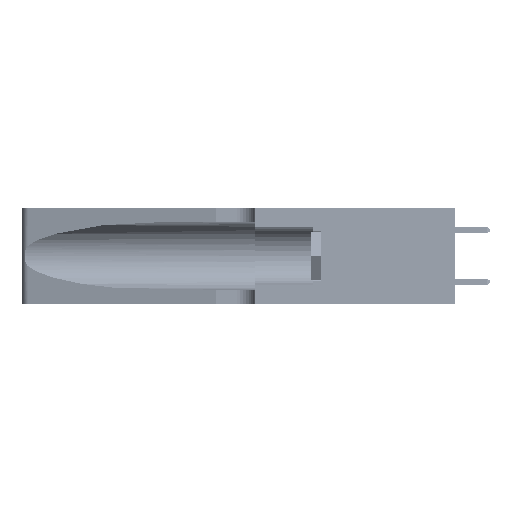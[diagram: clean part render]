
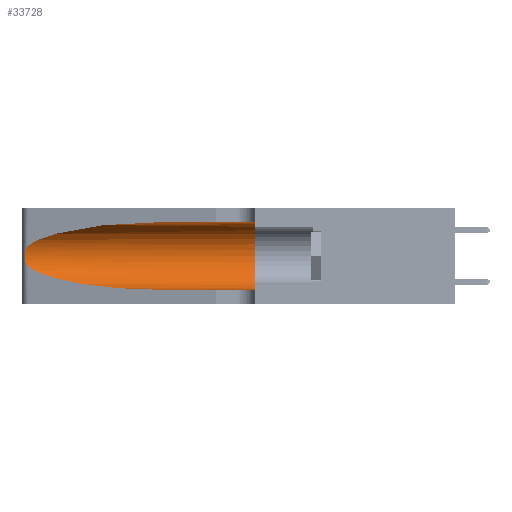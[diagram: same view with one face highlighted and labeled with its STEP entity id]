
A CAD part, left-side view. The second image highlights one B-rep face of the part: STEP entity #33728.
In plain terms, the highlighted cylindrical face has radius 3.308 mm (diameter 6.617 mm), a partial arc.
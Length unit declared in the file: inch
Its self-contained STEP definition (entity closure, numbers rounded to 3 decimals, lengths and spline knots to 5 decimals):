
#523 = VERTEX_POINT ( 'NONE', #7090 ) ;
#2039 = VERTEX_POINT ( 'NONE', #13384 ) ;
#2302 = VERTEX_POINT ( 'NONE', #48875 ) ;
#2403 = VECTOR ( 'NONE', #39100, 39.37008 ) ;
#3396 = LINE ( 'NONE', #21980, #17135 ) ;
#3776 = ORIENTED_EDGE ( 'NONE', *, *, #5392, .T. ) ;
#4815 = CYLINDRICAL_SURFACE ( 'NONE', #41524, 0.13025 ) ;
#5392 = EDGE_CURVE ( 'NONE', #2302, #32435, #41210, .T. ) ;
#6046 = CARTESIAN_POINT ( 'NONE',  ( 0.25639, 1.23186, 0.15144 ) ) ;
#7090 = CARTESIAN_POINT ( 'NONE',  ( 0.1305, 0.35, 0.31525 ) ) ;
#7430 = FACE_OUTER_BOUND ( 'NONE', #9912, .T. ) ;
#9493 = DIRECTION ( 'NONE',  ( 0., 1., 0. ) ) ;
#9912 = EDGE_LOOP ( 'NONE', ( #3776, #40965, #29007, #22652, #28667, #22535 ) ) ;
#10373 = CARTESIAN_POINT ( 'NONE',  ( 0.25639, 1.23184, 0.21858 ) ) ;
#11525 = CARTESIAN_POINT ( 'NONE',  ( 0.1305, 1.61858, 0.185 ) ) ;
#13384 = CARTESIAN_POINT ( 'NONE',  ( 0.25487, 1.22718, 0.14631 ) ) ;
#14968 = VERTEX_POINT ( 'NONE', #16529 ) ;
#15858 = CARTESIAN_POINT ( 'NONE',  ( 0.25487, 1.22718, 0.22369 ) ) ;
#16148 = DIRECTION ( 'NONE',  ( 0., 0., -1. ) ) ;
#16529 = CARTESIAN_POINT ( 'NONE',  ( 0.1305, 0.72297, 0.05475 ) ) ;
#17135 = VECTOR ( 'NONE', #51226, 39.37008 ) ;
#18292 = CARTESIAN_POINT ( 'NONE',  ( 0.25787, 1.23484, 0.2124 ) ) ;
#19939 = CIRCLE ( 'NONE', #35806, 0.13025 ) ;
#20178 = DIRECTION ( 'NONE',  ( 0., -1., 0. ) ) ;
#20579 = EDGE_CURVE ( 'NONE', #523, #42162, #19939, .T. ) ;
#21980 = CARTESIAN_POINT ( 'NONE',  ( 0.1305, 1.61858, 0.05475 ) ) ;
#22315 = CARTESIAN_POINT ( 'NONE',  ( 0.26018, 1.23835, 0.19895 ) ) ;
#22503 = CARTESIAN_POINT ( 'NONE',  ( 0.26017, 1.23833, 0.17102 ) ) ;
#22535 = ORIENTED_EDGE ( 'NONE', *, *, #44434, .F. ) ;
#22652 = ORIENTED_EDGE ( 'NONE', *, *, #53370, .T. ) ;
#23007 = CARTESIAN_POINT ( 'NONE',  ( 0.1305, 1.61858, 0.31525 ) ) ;
#24671 = CARTESIAN_POINT ( 'NONE',  ( 0.2373, 1.15595, 0.28018 ) ) ;
#24755 = CARTESIAN_POINT ( 'NONE',  ( 0.1305, 0.72297, 0.05475 ) ) ;
#25222 = CARTESIAN_POINT ( 'NONE',  ( 0.25487, 1.22718, 0.22369 ) ) ;
#26155 = CARTESIAN_POINT ( 'NONE',  ( 0.1305, 0.35, 0.185 ) ) ;
#26869 = CARTESIAN_POINT ( 'NONE',  ( 0.25856, 1.23593, 0.16098 ) ) ;
#28667 = ORIENTED_EDGE ( 'NONE', *, *, #20579, .F. ) ;
#29007 = ORIENTED_EDGE ( 'NONE', *, *, #31150, .T. ) ;
#31076 = CARTESIAN_POINT ( 'NONE',  ( 0.26075, 1.23896, 0.178 ) ) ;
#31150 = EDGE_CURVE ( 'NONE', #2039, #14968, #37190, .T. ) ;
#32435 = VERTEX_POINT ( 'NONE', #15858 ) ;
#33110 = CARTESIAN_POINT ( 'NONE',  ( 0.18966, 0.96281, 0.31525 ) ) ;
#33645 = CARTESIAN_POINT ( 'NONE',  ( 0.1305, 0.72297, 0.31525 ) ) ;
#33728 = ADVANCED_FACE ( 'NONE', ( #7430 ), #4815, .F. ) ;
#34932 = CARTESIAN_POINT ( 'NONE',  ( 0.25854, 1.2359, 0.20912 ) ) ;
#35287 = CARTESIAN_POINT ( 'NONE',  ( 0.25555, 1.22993, 0.14849 ) ) ;
#35806 = AXIS2_PLACEMENT_3D ( 'NONE', #26155, #9493, #38766 ) ;
#37190 =( BOUNDED_CURVE ( )  B_SPLINE_CURVE ( 3, ( #37193, #41573, #53659, #24755 ),
 .UNSPECIFIED., .F., .F. ) 
 B_SPLINE_CURVE_WITH_KNOTS ( ( 4, 4 ),
 ( 3.44316, 4.71239 ),
 .UNSPECIFIED. ) 
 CURVE ( )  GEOMETRIC_REPRESENTATION_ITEM ( )  RATIONAL_B_SPLINE_CURVE ( ( 1., 0.87, 0.87, 1. ) ) 
 REPRESENTATION_ITEM ( '' )  );
#37193 = CARTESIAN_POINT ( 'NONE',  ( 0.25487, 1.22718, 0.14631 ) ) ;
#38418 = EDGE_CURVE ( 'NONE', #32435, #2039, #42881, .T. ) ;
#38766 = DIRECTION ( 'NONE',  ( 0., 0., 1. ) ) ;
#39100 = DIRECTION ( 'NONE',  ( 0., -1., 0. ) ) ;
#40965 = ORIENTED_EDGE ( 'NONE', *, *, #38418, .T. ) ;
#41210 =( BOUNDED_CURVE ( )  B_SPLINE_CURVE ( 3, ( #33645, #33110, #24671, #25222 ),
 .UNSPECIFIED., .F., .F. ) 
 B_SPLINE_CURVE_WITH_KNOTS ( ( 4, 4 ),
 ( 1.5708, 2.84003 ),
 .UNSPECIFIED. ) 
 CURVE ( )  GEOMETRIC_REPRESENTATION_ITEM ( )  RATIONAL_B_SPLINE_CURVE ( ( 1., 0.87, 0.87, 1. ) ) 
 REPRESENTATION_ITEM ( '' )  );
#41524 = AXIS2_PLACEMENT_3D ( 'NONE', #11525, #20178, #16148 ) ;
#41573 = CARTESIAN_POINT ( 'NONE',  ( 0.2373, 1.15595, 0.08982 ) ) ;
#42162 = VERTEX_POINT ( 'NONE', #52659 ) ;
#42881 = B_SPLINE_CURVE_WITH_KNOTS ( 'NONE', 3,
 ( #51938, #47376, #10373, #18292, #34932, #22315, #48099, #31076, #22503, #26869, #51750, #6046, #35287, #43684 ),
 .UNSPECIFIED., .F., .F.,
 ( 4, 2, 2, 2, 2, 2, 4 ),
 ( 0., 0.00027, 0.00053, 0.00107, 0.0016, 0.00187, 0.00214 ),
 .UNSPECIFIED. ) ;
#43684 = CARTESIAN_POINT ( 'NONE',  ( 0.25487, 1.22718, 0.14631 ) ) ;
#44434 = EDGE_CURVE ( 'NONE', #2302, #523, #50131, .T. ) ;
#47376 = CARTESIAN_POINT ( 'NONE',  ( 0.25555, 1.22994, 0.2215 ) ) ;
#48099 = CARTESIAN_POINT ( 'NONE',  ( 0.26075, 1.23896, 0.19203 ) ) ;
#48875 = CARTESIAN_POINT ( 'NONE',  ( 0.1305, 0.72297, 0.31525 ) ) ;
#50131 = LINE ( 'NONE', #23007, #2403 ) ;
#51226 = DIRECTION ( 'NONE',  ( 0., -1., 0. ) ) ;
#51750 = CARTESIAN_POINT ( 'NONE',  ( 0.25789, 1.23486, 0.15765 ) ) ;
#51938 = CARTESIAN_POINT ( 'NONE',  ( 0.25487, 1.22718, 0.22369 ) ) ;
#52659 = CARTESIAN_POINT ( 'NONE',  ( 0.1305, 0.35, 0.05475 ) ) ;
#53370 = EDGE_CURVE ( 'NONE', #14968, #42162, #3396, .T. ) ;
#53659 = CARTESIAN_POINT ( 'NONE',  ( 0.18966, 0.96281, 0.05475 ) ) ;
